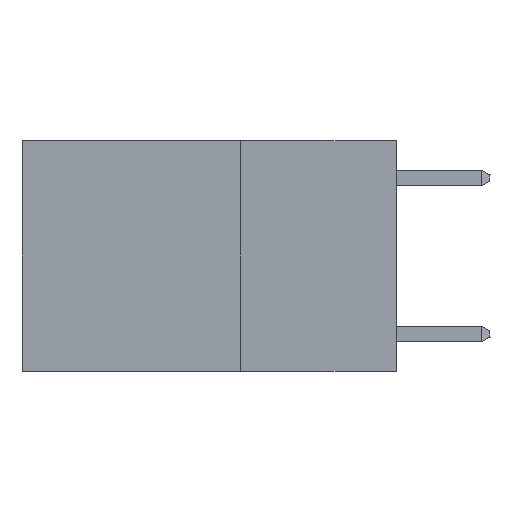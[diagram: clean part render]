
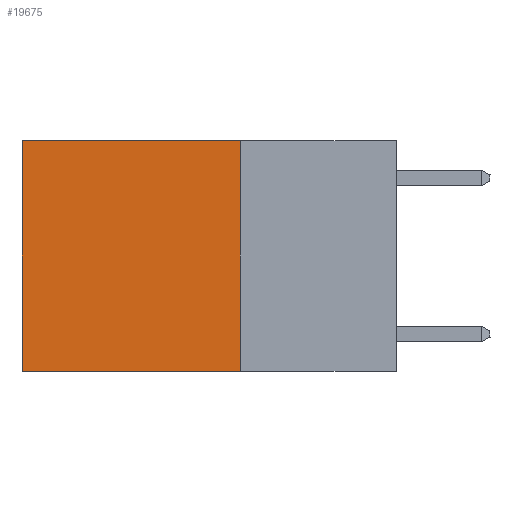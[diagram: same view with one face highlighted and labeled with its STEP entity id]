
A CAD part, left-side view. The second image highlights one B-rep face of the part: STEP entity #19675.
In plain terms, the highlighted planar face has unit normal (-1, 0, 0).
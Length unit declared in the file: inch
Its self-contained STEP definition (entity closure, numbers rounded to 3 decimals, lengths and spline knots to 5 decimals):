
#66 = EDGE_CURVE ( 'NONE', #23349, #25167, #17695, .T. ) ;
#1572 = EDGE_CURVE ( 'NONE', #8604, #23349, #22024, .T. ) ;
#1577 = EDGE_CURVE ( 'NONE', #8604, #6249, #7661, .T. ) ;
#1851 = VECTOR ( 'NONE', #13722, 39.37008 ) ;
#4703 = CARTESIAN_POINT ( 'NONE',  ( 0.2625, 0.6, 0. ) ) ;
#4881 = ORIENTED_EDGE ( 'NONE', *, *, #66, .T. ) ;
#5091 = DIRECTION ( 'NONE',  ( 0., 1., 0. ) ) ;
#5297 = CARTESIAN_POINT ( 'NONE',  ( 0.2625, 0.6, 0. ) ) ;
#5823 = DIRECTION ( 'NONE',  ( 1., 0., 0. ) ) ;
#6249 = VERTEX_POINT ( 'NONE', #11043 ) ;
#7661 = LINE ( 'NONE', #17597, #1851 ) ;
#7945 = ORIENTED_EDGE ( 'NONE', *, *, #1577, .F. ) ;
#8604 = VERTEX_POINT ( 'NONE', #18774 ) ;
#9635 = CARTESIAN_POINT ( 'NONE',  ( 0.2625, 0.25, 0. ) ) ;
#10278 = CARTESIAN_POINT ( 'NONE',  ( 0.2625, 0.6, -0.37 ) ) ;
#10854 = ORIENTED_EDGE ( 'NONE', *, *, #1572, .T. ) ;
#11043 = CARTESIAN_POINT ( 'NONE',  ( 0.2625, 0.25, -0.37 ) ) ;
#11480 = VECTOR ( 'NONE', #5091, 39.37008 ) ;
#12108 = CARTESIAN_POINT ( 'NONE',  ( 0.2625, 0.25, 0. ) ) ;
#12334 = EDGE_LOOP ( 'NONE', ( #4881, #20485, #7945, #10854 ) ) ;
#13343 = LINE ( 'NONE', #25049, #11480 ) ;
#13722 = DIRECTION ( 'NONE',  ( 0., 0., -1. ) ) ;
#13818 = DIRECTION ( 'NONE',  ( 0., 0., -1. ) ) ;
#15806 = DIRECTION ( 'NONE',  ( 0., 1., 0. ) ) ;
#17396 = AXIS2_PLACEMENT_3D ( 'NONE', #12108, #5823, #13818 ) ;
#17597 = CARTESIAN_POINT ( 'NONE',  ( 0.2625, 0.25, 0. ) ) ;
#17695 = LINE ( 'NONE', #5297, #18939 ) ;
#18547 = VECTOR ( 'NONE', #15806, 39.37008 ) ;
#18774 = CARTESIAN_POINT ( 'NONE',  ( 0.2625, 0.25, 0. ) ) ;
#18939 = VECTOR ( 'NONE', #19381, 39.37008 ) ;
#19381 = DIRECTION ( 'NONE',  ( 0., 0., -1. ) ) ;
#19675 = ADVANCED_FACE ( 'NONE', ( #23685 ), #22122, .F. ) ;
#20485 = ORIENTED_EDGE ( 'NONE', *, *, #23416, .F. ) ;
#22024 = LINE ( 'NONE', #9635, #18547 ) ;
#22122 = PLANE ( 'NONE',  #17396 ) ;
#23349 = VERTEX_POINT ( 'NONE', #4703 ) ;
#23416 = EDGE_CURVE ( 'NONE', #6249, #25167, #13343, .T. ) ;
#23685 = FACE_OUTER_BOUND ( 'NONE', #12334, .T. ) ;
#25049 = CARTESIAN_POINT ( 'NONE',  ( 0.2625, 0.25, -0.37 ) ) ;
#25167 = VERTEX_POINT ( 'NONE', #10278 ) ;
